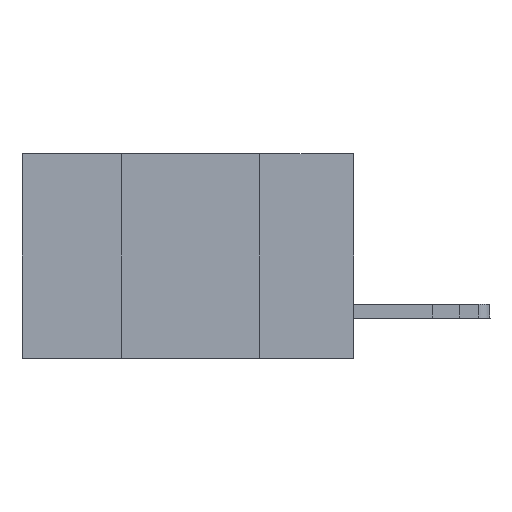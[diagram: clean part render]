
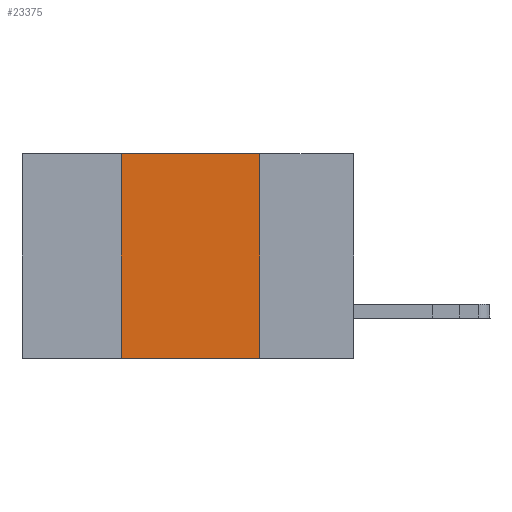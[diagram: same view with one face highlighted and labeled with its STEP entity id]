
A CAD part, left-side view. The second image highlights one B-rep face of the part: STEP entity #23375.
In plain terms, the highlighted planar face has unit normal (-1, 0, 0).
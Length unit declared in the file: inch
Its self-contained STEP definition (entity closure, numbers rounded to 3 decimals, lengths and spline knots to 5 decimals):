
#947 = EDGE_CURVE ( 'NONE', #8750, #9891, #11572, .T. ) ;
#1286 = FACE_OUTER_BOUND ( 'NONE', #11995, .T. ) ;
#1484 = DIRECTION ( 'NONE',  ( 1., 0., 0. ) ) ;
#1600 = CARTESIAN_POINT ( 'NONE',  ( 0., 0.6, 0. ) ) ;
#1644 = CARTESIAN_POINT ( 'NONE',  ( 0., 0.6, -0.37 ) ) ;
#3635 = CARTESIAN_POINT ( 'NONE',  ( 0., 0.17, 0. ) ) ;
#4227 = DIRECTION ( 'NONE',  ( 0., -1., 0. ) ) ;
#4917 = LINE ( 'NONE', #22896, #11387 ) ;
#4931 = CARTESIAN_POINT ( 'NONE',  ( 0., 0.17, -0.37 ) ) ;
#4975 = EDGE_CURVE ( 'NONE', #9547, #22140, #10701, .T. ) ;
#6802 = ORIENTED_EDGE ( 'NONE', *, *, #9966, .F. ) ;
#8750 = VERTEX_POINT ( 'NONE', #9294 ) ;
#9294 = CARTESIAN_POINT ( 'NONE',  ( 0., 0.42, -0.37 ) ) ;
#9547 = VERTEX_POINT ( 'NONE', #19761 ) ;
#9891 = VERTEX_POINT ( 'NONE', #4931 ) ;
#9966 = EDGE_CURVE ( 'NONE', #8750, #9547, #4917, .T. ) ;
#10363 = ORIENTED_EDGE ( 'NONE', *, *, #4975, .F. ) ;
#10701 = LINE ( 'NONE', #1600, #21166 ) ;
#11387 = VECTOR ( 'NONE', #13108, 39.37008 ) ;
#11572 = LINE ( 'NONE', #1644, #12825 ) ;
#11995 = EDGE_LOOP ( 'NONE', ( #24817, #10363, #6802, #15166 ) ) ;
#12825 = VECTOR ( 'NONE', #15141, 39.37008 ) ;
#13108 = DIRECTION ( 'NONE',  ( 0., 0., 1. ) ) ;
#15141 = DIRECTION ( 'NONE',  ( 0., -1., 0. ) ) ;
#15166 = ORIENTED_EDGE ( 'NONE', *, *, #947, .T. ) ;
#15324 = DIRECTION ( 'NONE',  ( 0., 0., -1. ) ) ;
#15460 = DIRECTION ( 'NONE',  ( 0., 0., -1. ) ) ;
#15915 = EDGE_CURVE ( 'NONE', #22140, #9891, #16131, .T. ) ;
#16131 = LINE ( 'NONE', #3635, #20766 ) ;
#17462 = CARTESIAN_POINT ( 'NONE',  ( 0., 0.17, 0. ) ) ;
#19761 = CARTESIAN_POINT ( 'NONE',  ( 0., 0.42, 0. ) ) ;
#20766 = VECTOR ( 'NONE', #15460, 39.37008 ) ;
#21166 = VECTOR ( 'NONE', #4227, 39.37008 ) ;
#22140 = VERTEX_POINT ( 'NONE', #17462 ) ;
#22896 = CARTESIAN_POINT ( 'NONE',  ( 0., 0.42, 0. ) ) ;
#22946 = AXIS2_PLACEMENT_3D ( 'NONE', #25014, #1484, #15324 ) ;
#23125 = PLANE ( 'NONE',  #22946 ) ;
#23375 = ADVANCED_FACE ( 'NONE', ( #1286 ), #23125, .F. ) ;
#24817 = ORIENTED_EDGE ( 'NONE', *, *, #15915, .F. ) ;
#25014 = CARTESIAN_POINT ( 'NONE',  ( 0., 0.6, 0. ) ) ;
